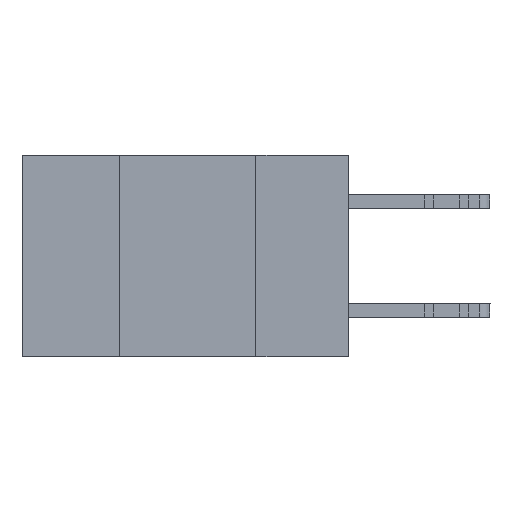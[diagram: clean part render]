
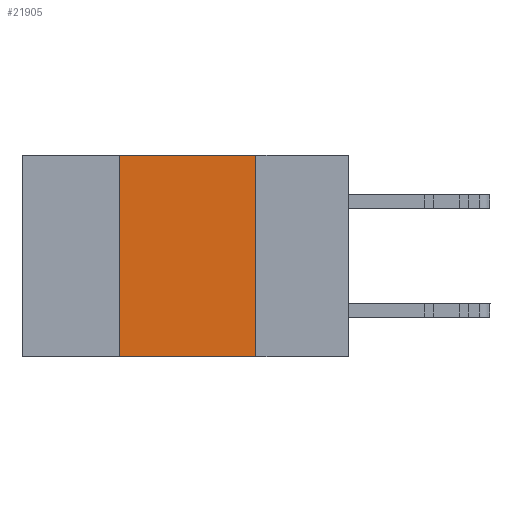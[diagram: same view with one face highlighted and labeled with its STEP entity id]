
A CAD part, left-side view. The second image highlights one B-rep face of the part: STEP entity #21905.
In plain terms, the highlighted planar face has unit normal (-1, 0, 0).
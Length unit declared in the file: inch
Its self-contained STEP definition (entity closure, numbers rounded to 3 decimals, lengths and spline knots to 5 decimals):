
#200 = ORIENTED_EDGE ( 'NONE', *, *, #13293, .F. ) ;
#694 = VERTEX_POINT ( 'NONE', #14052 ) ;
#729 = LINE ( 'NONE', #6935, #14696 ) ;
#2608 = LINE ( 'NONE', #14127, #17876 ) ;
#2928 = LINE ( 'NONE', #9622, #7597 ) ;
#4265 = PLANE ( 'NONE',  #16861 ) ;
#4474 = ORIENTED_EDGE ( 'NONE', *, *, #14607, .T. ) ;
#4841 = CARTESIAN_POINT ( 'NONE',  ( 0., 0.42, -0.37 ) ) ;
#5641 = ORIENTED_EDGE ( 'NONE', *, *, #9545, .F. ) ;
#6021 = FACE_OUTER_BOUND ( 'NONE', #17186, .T. ) ;
#6367 = DIRECTION ( 'NONE',  ( 0., 0., -1. ) ) ;
#6935 = CARTESIAN_POINT ( 'NONE',  ( 0., 0.6, -0.37 ) ) ;
#7597 = VECTOR ( 'NONE', #11602, 39.37008 ) ;
#8637 = VECTOR ( 'NONE', #21849, 39.37008 ) ;
#9545 = EDGE_CURVE ( 'NONE', #18675, #20313, #24566, .T. ) ;
#9622 = CARTESIAN_POINT ( 'NONE',  ( 0., 0.6, 0. ) ) ;
#11573 = VERTEX_POINT ( 'NONE', #4841 ) ;
#11602 = DIRECTION ( 'NONE',  ( 0., -1., 0. ) ) ;
#11901 = CARTESIAN_POINT ( 'NONE',  ( 0., 0.17, -0.37 ) ) ;
#13293 = EDGE_CURVE ( 'NONE', #694, #18675, #2928, .T. ) ;
#13393 = ORIENTED_EDGE ( 'NONE', *, *, #21845, .F. ) ;
#14017 = CARTESIAN_POINT ( 'NONE',  ( 0., 0.17, -0.37 ) ) ;
#14052 = CARTESIAN_POINT ( 'NONE',  ( 0., 0.42, 0. ) ) ;
#14127 = CARTESIAN_POINT ( 'NONE',  ( 0., 0.42, -0.37 ) ) ;
#14607 = EDGE_CURVE ( 'NONE', #11573, #20313, #729, .T. ) ;
#14696 = VECTOR ( 'NONE', #18867, 39.37008 ) ;
#16131 = DIRECTION ( 'NONE',  ( 0., 0., 1. ) ) ;
#16310 = CARTESIAN_POINT ( 'NONE',  ( 0., 0.6, 0. ) ) ;
#16861 = AXIS2_PLACEMENT_3D ( 'NONE', #16310, #18296, #6367 ) ;
#17186 = EDGE_LOOP ( 'NONE', ( #5641, #200, #13393, #4474 ) ) ;
#17876 = VECTOR ( 'NONE', #16131, 39.37008 ) ;
#18296 = DIRECTION ( 'NONE',  ( 1., 0., 0. ) ) ;
#18675 = VERTEX_POINT ( 'NONE', #23344 ) ;
#18867 = DIRECTION ( 'NONE',  ( 0., -1., 0. ) ) ;
#20313 = VERTEX_POINT ( 'NONE', #14017 ) ;
#21845 = EDGE_CURVE ( 'NONE', #11573, #694, #2608, .T. ) ;
#21849 = DIRECTION ( 'NONE',  ( 0., 0., -1. ) ) ;
#21905 = ADVANCED_FACE ( 'NONE', ( #6021 ), #4265, .F. ) ;
#23344 = CARTESIAN_POINT ( 'NONE',  ( 0., 0.17, 0. ) ) ;
#24566 = LINE ( 'NONE', #11901, #8637 ) ;
